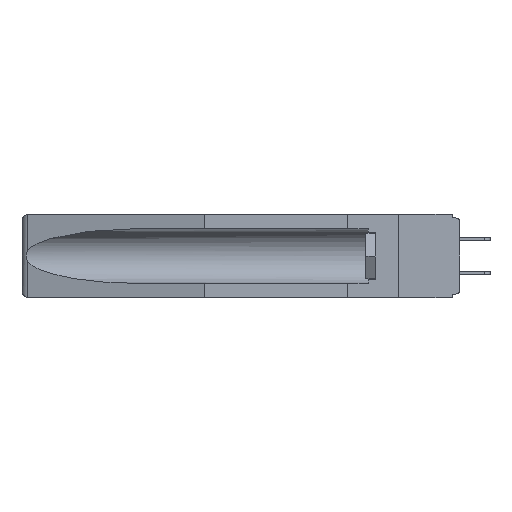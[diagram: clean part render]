
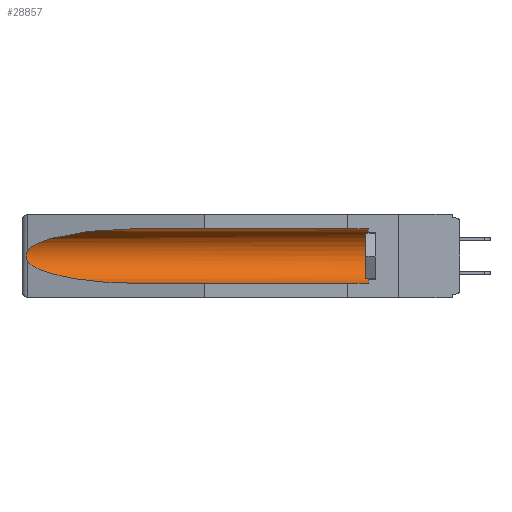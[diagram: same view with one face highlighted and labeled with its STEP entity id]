
A CAD part, left-side view. The second image highlights one B-rep face of the part: STEP entity #28857.
In plain terms, the highlighted cylindrical face has radius 2.857 mm (diameter 5.715 mm), a partial arc.
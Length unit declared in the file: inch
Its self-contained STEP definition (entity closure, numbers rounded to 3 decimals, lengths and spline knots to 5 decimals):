
#812 = CARTESIAN_POINT ( 'NONE',  ( 0.155, -0.30754, -0.284 ) ) ;
#1418 = LINE ( 'NONE', #27044, #20397 ) ;
#1545 = FACE_OUTER_BOUND ( 'NONE', #9867, .T. ) ;
#1806 = CARTESIAN_POINT ( 'NONE',  ( 0.2675, 1.53308, -0.17534 ) ) ;
#2343 = CARTESIAN_POINT ( 'NONE',  ( 0.155, 1.07973, -0.284 ) ) ;
#2838 = DIRECTION ( 'NONE',  ( 0., 1., 0. ) ) ;
#4357 = CARTESIAN_POINT ( 'NONE',  ( 0.26537, 1.52718, -0.14972 ) ) ;
#4404 = CARTESIAN_POINT ( 'NONE',  ( 0.2673, 1.53269, -0.17917 ) ) ;
#4725 = CARTESIAN_POINT ( 'NONE',  ( 0.25451, 1.48313, -0.24835 ) ) ;
#4909 = DIRECTION ( 'NONE',  ( 0., 0., 1. ) ) ;
#5516 = CARTESIAN_POINT ( 'NONE',  ( 0.155, 0.126, -0.284 ) ) ;
#6063 =( BOUNDED_CURVE ( )  B_SPLINE_CURVE ( 3, ( #20303, #4725, #27817, #2343 ),
 .UNSPECIFIED., .F., .F. ) 
 B_SPLINE_CURVE_WITH_KNOTS ( ( 4, 4 ),
 ( 0.1948, 1.5708 ),
 .UNSPECIFIED. ) 
 CURVE ( )  GEOMETRIC_REPRESENTATION_ITEM ( )  RATIONAL_B_SPLINE_CURVE ( ( 1., 0.848, 0.848, 1. ) ) 
 REPRESENTATION_ITEM ( '' )  );
#7045 = CARTESIAN_POINT ( 'NONE',  ( 0.26537, 1.52718, -0.14972 ) ) ;
#7680 = CARTESIAN_POINT ( 'NONE',  ( 0.26597, 1.5296, -0.19026 ) ) ;
#8529 = B_SPLINE_CURVE_WITH_KNOTS ( 'NONE', 3,
 ( #20198, #14656, #12504, #17259, #25022, #1806, #4404, #19985, #7680, #23323 ),
 .UNSPECIFIED., .F., .F.,
 ( 4, 2, 2, 2, 4 ),
 ( 0., 0.00029, 0.00058, 0.00087, 0.00117 ),
 .UNSPECIFIED. ) ;
#9867 = EDGE_LOOP ( 'NONE', ( #29389, #32333, #16447, #30450, #19476, #15971 ) ) ;
#10546 = VERTEX_POINT ( 'NONE', #29971 ) ;
#11779 = CARTESIAN_POINT ( 'NONE',  ( 0.26537, 1.52718, -0.19328 ) ) ;
#11836 = VERTEX_POINT ( 'NONE', #5516 ) ;
#12403 = VERTEX_POINT ( 'NONE', #13675 ) ;
#12504 = CARTESIAN_POINT ( 'NONE',  ( 0.26654, 1.53092, -0.15636 ) ) ;
#13675 = CARTESIAN_POINT ( 'NONE',  ( 0.155, 0.126, -0.059 ) ) ;
#14112 = CARTESIAN_POINT ( 'NONE',  ( 0.155, 1.07973, -0.284 ) ) ;
#14560 = VERTEX_POINT ( 'NONE', #11779 ) ;
#14656 = CARTESIAN_POINT ( 'NONE',  ( 0.26597, 1.52961, -0.15275 ) ) ;
#14935 = CARTESIAN_POINT ( 'NONE',  ( 0.155, 1.07973, -0.059 ) ) ;
#15190 = VERTEX_POINT ( 'NONE', #7045 ) ;
#15971 = ORIENTED_EDGE ( 'NONE', *, *, #25126, .T. ) ;
#16447 = ORIENTED_EDGE ( 'NONE', *, *, #24240, .T. ) ;
#17070 = VECTOR ( 'NONE', #2838, 39.37008 ) ;
#17259 = CARTESIAN_POINT ( 'NONE',  ( 0.2673, 1.5327, -0.16383 ) ) ;
#17573 = DIRECTION ( 'NONE',  ( 0., -1., 0. ) ) ;
#17625 = EDGE_CURVE ( 'NONE', #11836, #12403, #26646, .T. ) ;
#19308 = DIRECTION ( 'NONE',  ( 0., 1., 0. ) ) ;
#19476 = ORIENTED_EDGE ( 'NONE', *, *, #17625, .T. ) ;
#19827 = CARTESIAN_POINT ( 'NONE',  ( 0.21114, 1.30732, -0.059 ) ) ;
#19985 = CARTESIAN_POINT ( 'NONE',  ( 0.26655, 1.53094, -0.18657 ) ) ;
#20050 = CARTESIAN_POINT ( 'NONE',  ( 0.25451, 1.48313, -0.09465 ) ) ;
#20198 = CARTESIAN_POINT ( 'NONE',  ( 0.26537, 1.52718, -0.14972 ) ) ;
#20303 = CARTESIAN_POINT ( 'NONE',  ( 0.26537, 1.52718, -0.19328 ) ) ;
#20397 = VECTOR ( 'NONE', #19308, 39.37008 ) ;
#22104 = EDGE_CURVE ( 'NONE', #15190, #14560, #8529, .T. ) ;
#22555 = CARTESIAN_POINT ( 'NONE',  ( 0.155, 0.126, -0.1715 ) ) ;
#23323 = CARTESIAN_POINT ( 'NONE',  ( 0.26537, 1.52718, -0.19328 ) ) ;
#23801 = EDGE_CURVE ( 'NONE', #11836, #29343, #23920, .T. ) ;
#23920 = LINE ( 'NONE', #812, #17070 ) ;
#24032 =( BOUNDED_CURVE ( )  B_SPLINE_CURVE ( 3, ( #14935, #19827, #20050, #4357 ),
 .UNSPECIFIED., .F., .F. ) 
 B_SPLINE_CURVE_WITH_KNOTS ( ( 4, 4 ),
 ( 4.71239, 6.08839 ),
 .UNSPECIFIED. ) 
 CURVE ( )  GEOMETRIC_REPRESENTATION_ITEM ( )  RATIONAL_B_SPLINE_CURVE ( ( 1., 0.848, 0.848, 1. ) ) 
 REPRESENTATION_ITEM ( '' )  );
#24240 = EDGE_CURVE ( 'NONE', #14560, #29343, #6063, .T. ) ;
#25022 = CARTESIAN_POINT ( 'NONE',  ( 0.2675, 1.53308, -0.16763 ) ) ;
#25126 = EDGE_CURVE ( 'NONE', #12403, #10546, #1418, .T. ) ;
#25806 = EDGE_CURVE ( 'NONE', #10546, #15190, #24032, .T. ) ;
#26165 = CYLINDRICAL_SURFACE ( 'NONE', #27825, 0.1125 ) ;
#26646 = CIRCLE ( 'NONE', #27731, 0.1125 ) ;
#27044 = CARTESIAN_POINT ( 'NONE',  ( 0.155, -0.30754, -0.059 ) ) ;
#27731 = AXIS2_PLACEMENT_3D ( 'NONE', #22555, #17573, #30404 ) ;
#27817 = CARTESIAN_POINT ( 'NONE',  ( 0.21114, 1.30732, -0.284 ) ) ;
#27825 = AXIS2_PLACEMENT_3D ( 'NONE', #28211, #33383, #4909 ) ;
#28211 = CARTESIAN_POINT ( 'NONE',  ( 0.155, -0.30754, -0.1715 ) ) ;
#28857 = ADVANCED_FACE ( 'NONE', ( #1545 ), #26165, .F. ) ;
#29343 = VERTEX_POINT ( 'NONE', #14112 ) ;
#29389 = ORIENTED_EDGE ( 'NONE', *, *, #25806, .T. ) ;
#29971 = CARTESIAN_POINT ( 'NONE',  ( 0.155, 1.07973, -0.059 ) ) ;
#30404 = DIRECTION ( 'NONE',  ( 0., 0., 1. ) ) ;
#30450 = ORIENTED_EDGE ( 'NONE', *, *, #23801, .F. ) ;
#32333 = ORIENTED_EDGE ( 'NONE', *, *, #22104, .T. ) ;
#33383 = DIRECTION ( 'NONE',  ( 0., 1., 0. ) ) ;
